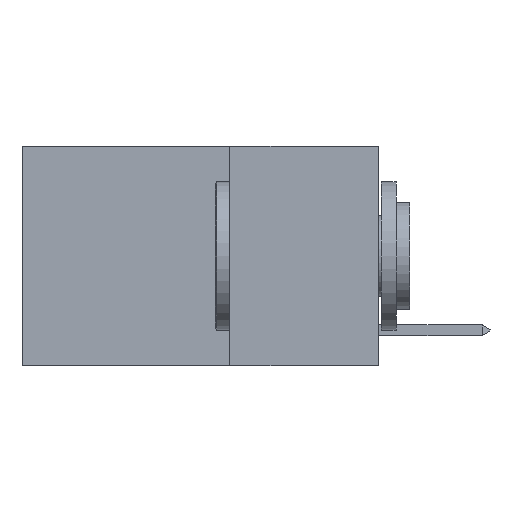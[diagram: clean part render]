
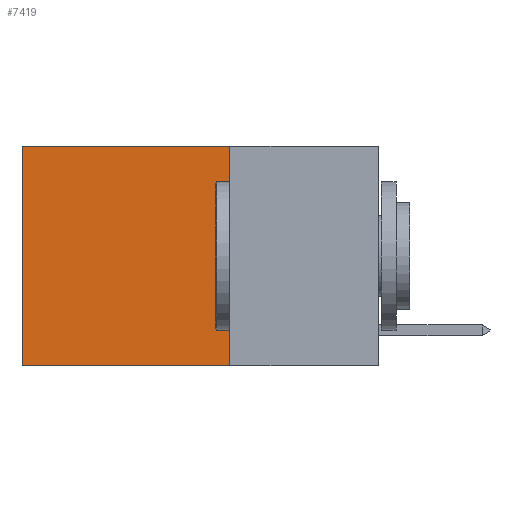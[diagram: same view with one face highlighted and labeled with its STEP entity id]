
A CAD part, left-side view. The second image highlights one B-rep face of the part: STEP entity #7419.
In plain terms, the highlighted planar face has unit normal (-1, 0, 0).
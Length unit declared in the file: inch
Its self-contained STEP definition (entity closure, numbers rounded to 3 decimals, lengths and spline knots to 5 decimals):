
#1319 = CARTESIAN_POINT ( 'NONE',  ( 0.2625, 0.25, -0.37 ) ) ;
#1438 = LINE ( 'NONE', #26386, #11413 ) ;
#1763 = VECTOR ( 'NONE', #7728, 39.37008 ) ;
#2755 = ORIENTED_EDGE ( 'NONE', *, *, #6479, .F. ) ;
#2960 = EDGE_CURVE ( 'NONE', #19149, #25465, #13091, .T. ) ;
#3147 = DIRECTION ( 'NONE',  ( 0., 0., -1. ) ) ;
#3225 = EDGE_LOOP ( 'NONE', ( #26025, #20742, #2755, #23832 ) ) ;
#3253 = LINE ( 'NONE', #13775, #25077 ) ;
#3753 = CARTESIAN_POINT ( 'NONE',  ( 0.2625, 0.25, 0. ) ) ;
#3779 = VECTOR ( 'NONE', #22693, 39.37008 ) ;
#5337 = CARTESIAN_POINT ( 'NONE',  ( 0.2625, 0.25, -0.37 ) ) ;
#5397 = DIRECTION ( 'NONE',  ( 0., 1., 0. ) ) ;
#6104 = FACE_OUTER_BOUND ( 'NONE', #3225, .T. ) ;
#6479 = EDGE_CURVE ( 'NONE', #26129, #19149, #1438, .T. ) ;
#7419 = ADVANCED_FACE ( 'NONE', ( #6104 ), #20698, .F. ) ;
#7728 = DIRECTION ( 'NONE',  ( 0., 1., 0. ) ) ;
#8035 = DIRECTION ( 'NONE',  ( 1., 0., 0. ) ) ;
#10404 = CARTESIAN_POINT ( 'NONE',  ( 0.2625, 0.6, 0. ) ) ;
#11413 = VECTOR ( 'NONE', #3147, 39.37008 ) ;
#13091 = LINE ( 'NONE', #1319, #1763 ) ;
#13775 = CARTESIAN_POINT ( 'NONE',  ( 0.2625, 0.25, 0. ) ) ;
#15155 = CARTESIAN_POINT ( 'NONE',  ( 0.2625, 0.6, -0.37 ) ) ;
#19149 = VERTEX_POINT ( 'NONE', #5337 ) ;
#20698 = PLANE ( 'NONE',  #24490 ) ;
#20742 = ORIENTED_EDGE ( 'NONE', *, *, #2960, .F. ) ;
#20831 = VERTEX_POINT ( 'NONE', #10404 ) ;
#21769 = EDGE_CURVE ( 'NONE', #20831, #25465, #25573, .T. ) ;
#22693 = DIRECTION ( 'NONE',  ( 0., 0., -1. ) ) ;
#22826 = DIRECTION ( 'NONE',  ( 0., 0., -1. ) ) ;
#23527 = CARTESIAN_POINT ( 'NONE',  ( 0.2625, 0.25, 0. ) ) ;
#23832 = ORIENTED_EDGE ( 'NONE', *, *, #25722, .T. ) ;
#24490 = AXIS2_PLACEMENT_3D ( 'NONE', #3753, #8035, #22826 ) ;
#25077 = VECTOR ( 'NONE', #5397, 39.37008 ) ;
#25465 = VERTEX_POINT ( 'NONE', #15155 ) ;
#25573 = LINE ( 'NONE', #26746, #3779 ) ;
#25722 = EDGE_CURVE ( 'NONE', #26129, #20831, #3253, .T. ) ;
#26025 = ORIENTED_EDGE ( 'NONE', *, *, #21769, .T. ) ;
#26129 = VERTEX_POINT ( 'NONE', #23527 ) ;
#26386 = CARTESIAN_POINT ( 'NONE',  ( 0.2625, 0.25, 0. ) ) ;
#26746 = CARTESIAN_POINT ( 'NONE',  ( 0.2625, 0.6, 0. ) ) ;
